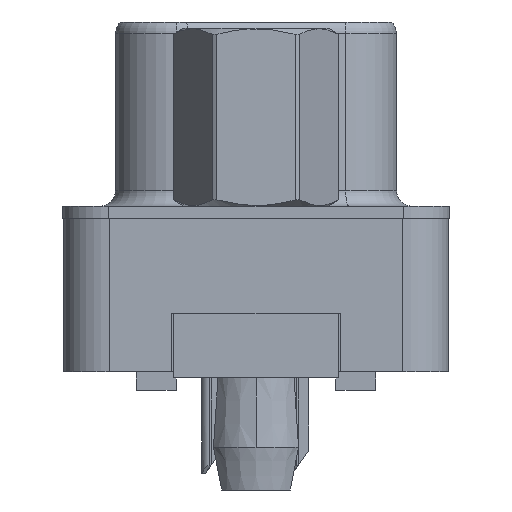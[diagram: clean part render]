
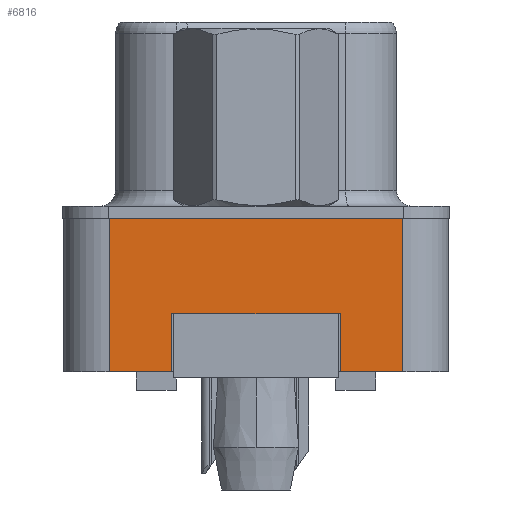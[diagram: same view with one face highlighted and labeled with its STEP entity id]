
A CAD part, left-side view. The second image highlights one B-rep face of the part: STEP entity #6816.
In plain terms, the highlighted planar face has unit normal (-1, 0, 0).
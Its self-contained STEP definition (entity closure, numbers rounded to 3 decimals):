
#424 = CARTESIAN_POINT ( 'NONE',  ( -3., -4.775, -5. ) ) ;
#1187 = VECTOR ( 'NONE', #15669, 1000. ) ;
#1384 = VERTEX_POINT ( 'NONE', #10576 ) ;
#2948 = CARTESIAN_POINT ( 'NONE',  ( -3., 2.75, -3.1 ) ) ;
#3393 = CARTESIAN_POINT ( 'NONE',  ( -3., -4.775, 0. ) ) ;
#4914 = LINE ( 'NONE', #24089, #8073 ) ;
#5081 = LINE ( 'NONE', #2948, #10958 ) ;
#5338 = LINE ( 'NONE', #9558, #15228 ) ;
#5391 = LINE ( 'NONE', #3393, #27627 ) ;
#5432 = EDGE_CURVE ( 'NONE', #8320, #24057, #18085, .T. ) ;
#5992 = DIRECTION ( 'NONE',  ( 0., 0., -1. ) ) ;
#6816 = ADVANCED_FACE ( 'NONE', ( #7207 ), #15808, .T. ) ;
#7037 = EDGE_LOOP ( 'NONE', ( #21802, #20053, #13966, #8740, #10929, #18895, #11380, #24911 ) ) ;
#7207 = FACE_OUTER_BOUND ( 'NONE', #7037, .T. ) ;
#7293 = EDGE_CURVE ( 'NONE', #27562, #16027, #4914, .T. ) ;
#7645 = CARTESIAN_POINT ( 'NONE',  ( -3., -4.775, -5. ) ) ;
#8073 = VECTOR ( 'NONE', #24368, 1000. ) ;
#8320 = VERTEX_POINT ( 'NONE', #9351 ) ;
#8740 = ORIENTED_EDGE ( 'NONE', *, *, #19863, .F. ) ;
#9351 = CARTESIAN_POINT ( 'NONE',  ( -3., -2.75, -5. ) ) ;
#9558 = CARTESIAN_POINT ( 'NONE',  ( -3., -4.775, -5. ) ) ;
#9635 = EDGE_CURVE ( 'NONE', #1384, #8320, #10625, .T. ) ;
#10411 = CARTESIAN_POINT ( 'NONE',  ( -3., -4.775, 0. ) ) ;
#10576 = CARTESIAN_POINT ( 'NONE',  ( -3., -2.75, -3.1 ) ) ;
#10625 = LINE ( 'NONE', #16838, #22577 ) ;
#10929 = ORIENTED_EDGE ( 'NONE', *, *, #12791, .F. ) ;
#10958 = VECTOR ( 'NONE', #11555, 1000. ) ;
#11380 = ORIENTED_EDGE ( 'NONE', *, *, #7293, .F. ) ;
#11416 = CARTESIAN_POINT ( 'NONE',  ( -3., 4.775, -5. ) ) ;
#11435 = LINE ( 'NONE', #24402, #1187 ) ;
#11538 = DIRECTION ( 'NONE',  ( 0., 0., 1. ) ) ;
#11555 = DIRECTION ( 'NONE',  ( 0., 1., 0. ) ) ;
#11848 = CARTESIAN_POINT ( 'NONE',  ( -3., 2.75, -3.1 ) ) ;
#12155 = DIRECTION ( 'NONE',  ( 0., -1., 0. ) ) ;
#12791 = EDGE_CURVE ( 'NONE', #19626, #25319, #23955, .T. ) ;
#13077 = AXIS2_PLACEMENT_3D ( 'NONE', #424, #19891, #15389 ) ;
#13485 = VECTOR ( 'NONE', #12155, 1000. ) ;
#13692 = EDGE_CURVE ( 'NONE', #1384, #27562, #5081, .T. ) ;
#13966 = ORIENTED_EDGE ( 'NONE', *, *, #27054, .T. ) ;
#15131 = CARTESIAN_POINT ( 'NONE',  ( -3., 4.775, -5. ) ) ;
#15228 = VECTOR ( 'NONE', #11538, 1000. ) ;
#15373 = VERTEX_POINT ( 'NONE', #10411 ) ;
#15389 = DIRECTION ( 'NONE',  ( 0., 0., 1. ) ) ;
#15669 = DIRECTION ( 'NONE',  ( 0., -1., 0. ) ) ;
#15808 = PLANE ( 'NONE',  #13077 ) ;
#16027 = VERTEX_POINT ( 'NONE', #19950 ) ;
#16838 = CARTESIAN_POINT ( 'NONE',  ( -3., -2.75, -3.1 ) ) ;
#18085 = LINE ( 'NONE', #7645, #13485 ) ;
#18735 = CARTESIAN_POINT ( 'NONE',  ( -3., 4.775, 0. ) ) ;
#18895 = ORIENTED_EDGE ( 'NONE', *, *, #25166, .T. ) ;
#19524 = VECTOR ( 'NONE', #26516, 1000. ) ;
#19626 = VERTEX_POINT ( 'NONE', #15131 ) ;
#19863 = EDGE_CURVE ( 'NONE', #25319, #15373, #5391, .T. ) ;
#19891 = DIRECTION ( 'NONE',  ( -1., 0., 0. ) ) ;
#19950 = CARTESIAN_POINT ( 'NONE',  ( -3., 2.75, -5. ) ) ;
#20053 = ORIENTED_EDGE ( 'NONE', *, *, #5432, .T. ) ;
#21802 = ORIENTED_EDGE ( 'NONE', *, *, #9635, .T. ) ;
#22577 = VECTOR ( 'NONE', #5992, 1000. ) ;
#23955 = LINE ( 'NONE', #11416, #19524 ) ;
#24057 = VERTEX_POINT ( 'NONE', #25791 ) ;
#24089 = CARTESIAN_POINT ( 'NONE',  ( -3., 2.75, -3.1 ) ) ;
#24368 = DIRECTION ( 'NONE',  ( 0., 0., -1. ) ) ;
#24402 = CARTESIAN_POINT ( 'NONE',  ( -3., -4.775, -5. ) ) ;
#24911 = ORIENTED_EDGE ( 'NONE', *, *, #13692, .F. ) ;
#24978 = DIRECTION ( 'NONE',  ( 0., -1., 0. ) ) ;
#25166 = EDGE_CURVE ( 'NONE', #19626, #16027, #11435, .T. ) ;
#25319 = VERTEX_POINT ( 'NONE', #18735 ) ;
#25791 = CARTESIAN_POINT ( 'NONE',  ( -3., -4.775, -5. ) ) ;
#26516 = DIRECTION ( 'NONE',  ( 0., 0., 1. ) ) ;
#27054 = EDGE_CURVE ( 'NONE', #24057, #15373, #5338, .T. ) ;
#27562 = VERTEX_POINT ( 'NONE', #11848 ) ;
#27627 = VECTOR ( 'NONE', #24978, 1000. ) ;
